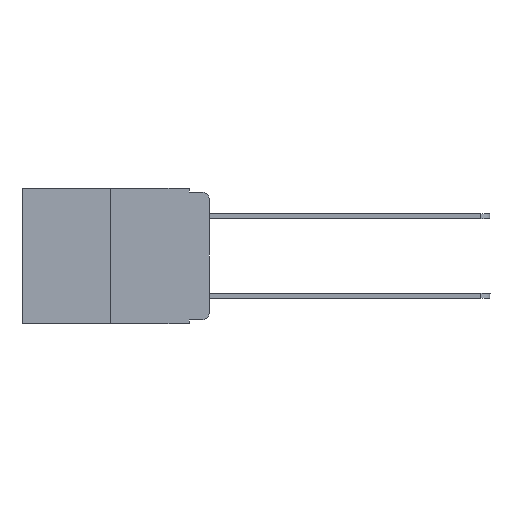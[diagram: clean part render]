
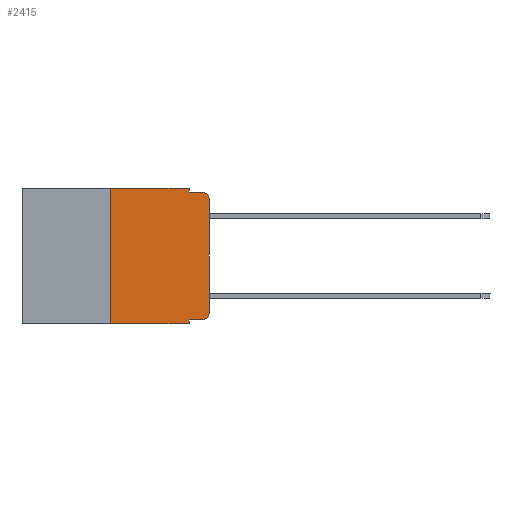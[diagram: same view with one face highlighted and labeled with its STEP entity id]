
A CAD part, left-side view. The second image highlights one B-rep face of the part: STEP entity #2415.
In plain terms, the highlighted planar face has unit normal (-1, 0, 0).
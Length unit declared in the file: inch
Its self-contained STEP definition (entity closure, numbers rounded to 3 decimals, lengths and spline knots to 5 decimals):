
#46 = EDGE_CURVE ( 'NONE', #3457, #3389, #3533, .T. ) ;
#62 = DIRECTION ( 'NONE',  ( 0., -1., 0. ) ) ;
#337 = ORIENTED_EDGE ( 'NONE', *, *, #1307, .T. ) ;
#502 = DIRECTION ( 'NONE',  ( 0., -1., 0. ) ) ;
#1048 = CARTESIAN_POINT ( 'NONE',  ( 0., 0.25, 0. ) ) ;
#1213 = CARTESIAN_POINT ( 'NONE',  ( 0., 0., -0.313 ) ) ;
#1307 = EDGE_CURVE ( 'NONE', #9223, #6050, #3923, .T. ) ;
#1340 = FACE_OUTER_BOUND ( 'NONE', #2582, .T. ) ;
#1407 = EDGE_CURVE ( 'NONE', #8818, #9223, #6437, .T. ) ;
#1547 = CARTESIAN_POINT ( 'NONE',  ( 0., 0., -0.03 ) ) ;
#1580 = VERTEX_POINT ( 'NONE', #6896 ) ;
#1641 = VERTEX_POINT ( 'NONE', #9318 ) ;
#1701 = CARTESIAN_POINT ( 'NONE',  ( 0., 0.051, 0. ) ) ;
#1859 = EDGE_CURVE ( 'NONE', #3937, #1641, #9626, .T. ) ;
#1923 = EDGE_CURVE ( 'NONE', #6402, #1641, #5451, .T. ) ;
#1989 = EDGE_CURVE ( 'NONE', #5813, #6402, #8286, .T. ) ;
#2184 = EDGE_CURVE ( 'NONE', #3457, #1580, #7826, .T. ) ;
#2229 = AXIS2_PLACEMENT_3D ( 'NONE', #5837, #8997, #9724 ) ;
#2387 = DIRECTION ( 'NONE',  ( 0., 0., -1. ) ) ;
#2415 = ADVANCED_FACE ( 'NONE', ( #1340 ), #3566, .F. ) ;
#2477 = CARTESIAN_POINT ( 'NONE',  ( 0., 0.051, -0.333 ) ) ;
#2582 = EDGE_LOOP ( 'NONE', ( #6185, #8168, #3121, #9695, #9519, #4856, #9635, #6018, #2917, #337 ) ) ;
#2808 = DIRECTION ( 'NONE',  ( -1., 0., 0. ) ) ;
#2917 = ORIENTED_EDGE ( 'NONE', *, *, #1407, .T. ) ;
#3121 = ORIENTED_EDGE ( 'NONE', *, *, #1923, .F. ) ;
#3368 = VECTOR ( 'NONE', #6629, 39.37008 ) ;
#3389 = VERTEX_POINT ( 'NONE', #3463 ) ;
#3457 = VERTEX_POINT ( 'NONE', #4664 ) ;
#3463 = CARTESIAN_POINT ( 'NONE',  ( 0., 0.051, -0.343 ) ) ;
#3533 = LINE ( 'NONE', #5697, #4830 ) ;
#3566 = PLANE ( 'NONE',  #2229 ) ;
#3680 = CARTESIAN_POINT ( 'NONE',  ( 0., 0.051, 0. ) ) ;
#3799 = EDGE_CURVE ( 'NONE', #8818, #3389, #5860, .T. ) ;
#3923 = CIRCLE ( 'NONE', #8208, 0.02 ) ;
#3937 = VERTEX_POINT ( 'NONE', #1547 ) ;
#3963 = CARTESIAN_POINT ( 'NONE',  ( 0., 0.051, -0.01 ) ) ;
#4060 = DIRECTION ( 'NONE',  ( 0., 0., 1. ) ) ;
#4265 = AXIS2_PLACEMENT_3D ( 'NONE', #9569, #2808, #8927 ) ;
#4279 = VECTOR ( 'NONE', #4060, 39.37008 ) ;
#4345 = CARTESIAN_POINT ( 'NONE',  ( 0., 0., 0. ) ) ;
#4664 = CARTESIAN_POINT ( 'NONE',  ( 0., 0.25, -0.343 ) ) ;
#4830 = VECTOR ( 'NONE', #8715, 39.37008 ) ;
#4856 = ORIENTED_EDGE ( 'NONE', *, *, #2184, .F. ) ;
#4923 = VECTOR ( 'NONE', #6795, 39.37008 ) ;
#4941 = CARTESIAN_POINT ( 'NONE',  ( 0., 0.051, -0.01 ) ) ;
#5300 = EDGE_CURVE ( 'NONE', #6050, #3937, #7396, .T. ) ;
#5451 = LINE ( 'NONE', #3963, #7092 ) ;
#5685 = VECTOR ( 'NONE', #2387, 39.37008 ) ;
#5697 = CARTESIAN_POINT ( 'NONE',  ( 0., 0.473, -0.343 ) ) ;
#5813 = VERTEX_POINT ( 'NONE', #9069 ) ;
#5837 = CARTESIAN_POINT ( 'NONE',  ( 0., 0.473, 0. ) ) ;
#5860 = LINE ( 'NONE', #3680, #4923 ) ;
#5933 = DIRECTION ( 'NONE',  ( -1., 0., 0. ) ) ;
#5988 = VECTOR ( 'NONE', #502, 39.37008 ) ;
#6018 = ORIENTED_EDGE ( 'NONE', *, *, #3799, .F. ) ;
#6050 = VERTEX_POINT ( 'NONE', #1213 ) ;
#6185 = ORIENTED_EDGE ( 'NONE', *, *, #5300, .T. ) ;
#6379 = CARTESIAN_POINT ( 'NONE',  ( 0., 0.02, -0.333 ) ) ;
#6402 = VERTEX_POINT ( 'NONE', #4941 ) ;
#6437 = LINE ( 'NONE', #9441, #5988 ) ;
#6629 = DIRECTION ( 'NONE',  ( 0., 0., 1. ) ) ;
#6795 = DIRECTION ( 'NONE',  ( 0., 0., -1. ) ) ;
#6896 = CARTESIAN_POINT ( 'NONE',  ( 0., 0.25, 0. ) ) ;
#7092 = VECTOR ( 'NONE', #9025, 39.37008 ) ;
#7396 = LINE ( 'NONE', #4345, #3368 ) ;
#7555 = VECTOR ( 'NONE', #62, 39.37008 ) ;
#7570 = LINE ( 'NONE', #7766, #7555 ) ;
#7766 = CARTESIAN_POINT ( 'NONE',  ( 0., 0.473, 0. ) ) ;
#7826 = LINE ( 'NONE', #1048, #4279 ) ;
#8168 = ORIENTED_EDGE ( 'NONE', *, *, #1859, .T. ) ;
#8208 = AXIS2_PLACEMENT_3D ( 'NONE', #8301, #5933, #8943 ) ;
#8286 = LINE ( 'NONE', #1701, #5685 ) ;
#8301 = CARTESIAN_POINT ( 'NONE',  ( 0., 0.02, -0.313 ) ) ;
#8715 = DIRECTION ( 'NONE',  ( 0., -1., 0. ) ) ;
#8818 = VERTEX_POINT ( 'NONE', #2477 ) ;
#8857 = EDGE_CURVE ( 'NONE', #1580, #5813, #7570, .T. ) ;
#8927 = DIRECTION ( 'NONE',  ( 0., 0., -1. ) ) ;
#8943 = DIRECTION ( 'NONE',  ( 0., 0., -1. ) ) ;
#8997 = DIRECTION ( 'NONE',  ( 1., 0., 0. ) ) ;
#9025 = DIRECTION ( 'NONE',  ( 0., -1., 0. ) ) ;
#9069 = CARTESIAN_POINT ( 'NONE',  ( 0., 0.051, 0. ) ) ;
#9223 = VERTEX_POINT ( 'NONE', #6379 ) ;
#9318 = CARTESIAN_POINT ( 'NONE',  ( 0., 0.02, -0.01 ) ) ;
#9441 = CARTESIAN_POINT ( 'NONE',  ( 0., 0.051, -0.333 ) ) ;
#9519 = ORIENTED_EDGE ( 'NONE', *, *, #8857, .F. ) ;
#9569 = CARTESIAN_POINT ( 'NONE',  ( 0., 0.02, -0.03 ) ) ;
#9626 = CIRCLE ( 'NONE', #4265, 0.02 ) ;
#9635 = ORIENTED_EDGE ( 'NONE', *, *, #46, .T. ) ;
#9695 = ORIENTED_EDGE ( 'NONE', *, *, #1989, .F. ) ;
#9724 = DIRECTION ( 'NONE',  ( 0., 0., -1. ) ) ;
